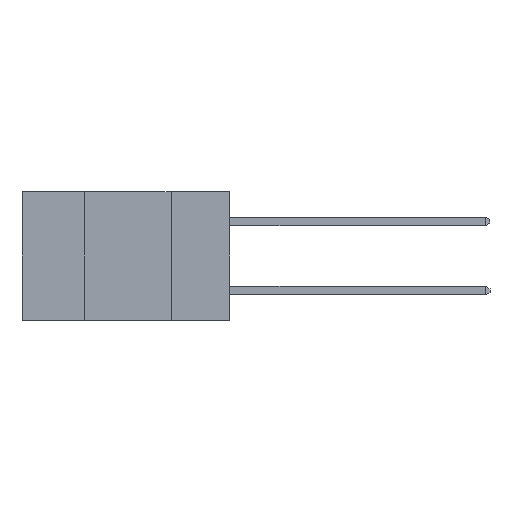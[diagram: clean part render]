
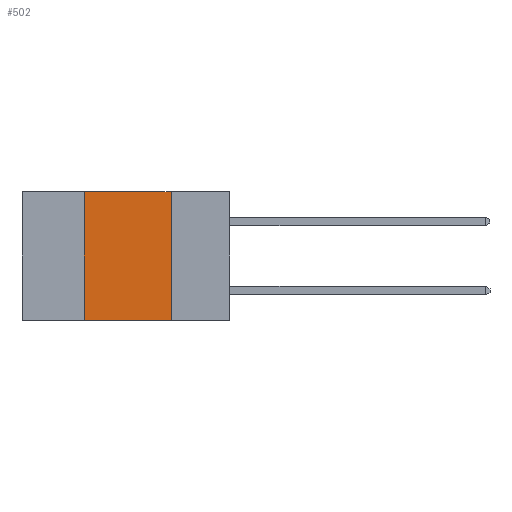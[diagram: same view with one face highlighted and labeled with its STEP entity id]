
A CAD part, left-side view. The second image highlights one B-rep face of the part: STEP entity #502.
In plain terms, the highlighted planar face has unit normal (-1, 0, 0).
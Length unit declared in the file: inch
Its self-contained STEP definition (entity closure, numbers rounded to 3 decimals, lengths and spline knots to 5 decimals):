
#478 = CARTESIAN_POINT ( 'NONE',  ( 0., 0.6, 0. ) ) ;
#502 = ADVANCED_FACE ( 'NONE', ( #4532 ), #2598, .F. ) ;
#649 = CARTESIAN_POINT ( 'NONE',  ( 0., 0.6, 0. ) ) ;
#769 = VERTEX_POINT ( 'NONE', #4097 ) ;
#850 = VERTEX_POINT ( 'NONE', #2030 ) ;
#1012 = DIRECTION ( 'NONE',  ( 0., -1., 0. ) ) ;
#1107 = CARTESIAN_POINT ( 'NONE',  ( 0., 0.17, -0.37 ) ) ;
#1252 = EDGE_CURVE ( 'NONE', #850, #7809, #6615, .T. ) ;
#1746 = EDGE_LOOP ( 'NONE', ( #3602, #8065, #6567, #3381 ) ) ;
#2030 = CARTESIAN_POINT ( 'NONE',  ( 0., 0.42, -0.37 ) ) ;
#2190 = VECTOR ( 'NONE', #1012, 39.37008 ) ;
#2415 = EDGE_CURVE ( 'NONE', #7809, #769, #5650, .T. ) ;
#2583 = DIRECTION ( 'NONE',  ( 1., 0., 0. ) ) ;
#2598 = PLANE ( 'NONE',  #4289 ) ;
#3053 = CARTESIAN_POINT ( 'NONE',  ( 0., 0.42, 0. ) ) ;
#3381 = ORIENTED_EDGE ( 'NONE', *, *, #7672, .T. ) ;
#3602 = ORIENTED_EDGE ( 'NONE', *, *, #4925, .F. ) ;
#4097 = CARTESIAN_POINT ( 'NONE',  ( 0., 0.17, 0. ) ) ;
#4289 = AXIS2_PLACEMENT_3D ( 'NONE', #478, #2583, #5022 ) ;
#4352 = VECTOR ( 'NONE', #8256, 39.37008 ) ;
#4532 = FACE_OUTER_BOUND ( 'NONE', #1746, .T. ) ;
#4825 = CARTESIAN_POINT ( 'NONE',  ( 0., 0.6, -0.37 ) ) ;
#4925 = EDGE_CURVE ( 'NONE', #769, #5838, #8230, .T. ) ;
#5022 = DIRECTION ( 'NONE',  ( 0., 0., -1. ) ) ;
#5234 = VECTOR ( 'NONE', #6635, 39.37008 ) ;
#5650 = LINE ( 'NONE', #649, #2190 ) ;
#5838 = VERTEX_POINT ( 'NONE', #1107 ) ;
#6365 = DIRECTION ( 'NONE',  ( 0., 0., -1. ) ) ;
#6529 = CARTESIAN_POINT ( 'NONE',  ( 0., 0.17, -0.37 ) ) ;
#6567 = ORIENTED_EDGE ( 'NONE', *, *, #1252, .F. ) ;
#6615 = LINE ( 'NONE', #7057, #5234 ) ;
#6635 = DIRECTION ( 'NONE',  ( 0., 0., 1. ) ) ;
#6748 = VECTOR ( 'NONE', #6365, 39.37008 ) ;
#7057 = CARTESIAN_POINT ( 'NONE',  ( 0., 0.42, -0.37 ) ) ;
#7442 = LINE ( 'NONE', #4825, #4352 ) ;
#7672 = EDGE_CURVE ( 'NONE', #850, #5838, #7442, .T. ) ;
#7809 = VERTEX_POINT ( 'NONE', #3053 ) ;
#8065 = ORIENTED_EDGE ( 'NONE', *, *, #2415, .F. ) ;
#8230 = LINE ( 'NONE', #6529, #6748 ) ;
#8256 = DIRECTION ( 'NONE',  ( 0., -1., 0. ) ) ;
